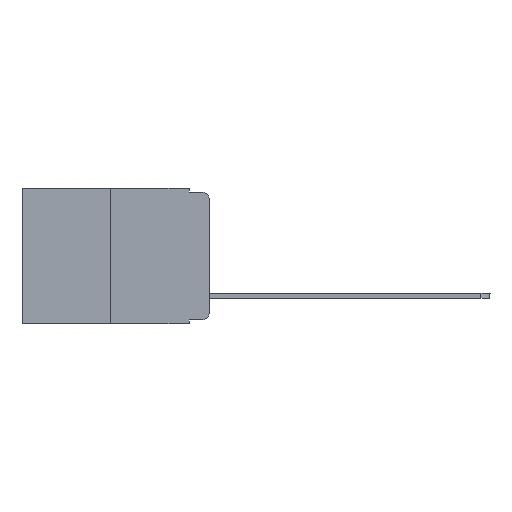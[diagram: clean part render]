
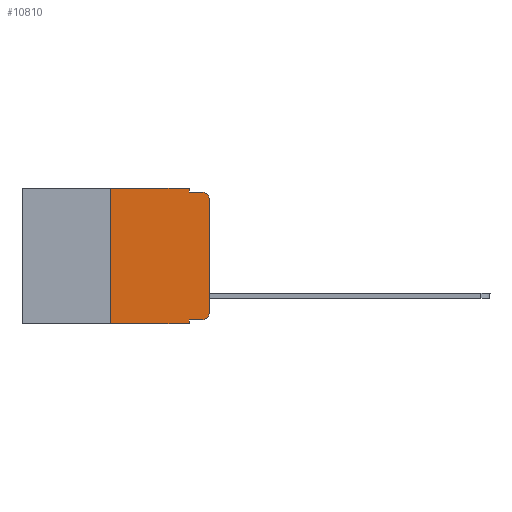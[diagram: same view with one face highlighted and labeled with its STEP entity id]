
A CAD part, left-side view. The second image highlights one B-rep face of the part: STEP entity #10810.
In plain terms, the highlighted planar face has unit normal (-1, 0, 0).
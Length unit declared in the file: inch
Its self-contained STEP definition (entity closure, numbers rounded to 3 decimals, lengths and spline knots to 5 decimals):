
#530 = EDGE_CURVE ( 'NONE', #2004, #8552, #6242, .T. ) ;
#583 = ORIENTED_EDGE ( 'NONE', *, *, #7575, .T. ) ;
#757 = VERTEX_POINT ( 'NONE', #7477 ) ;
#797 = CARTESIAN_POINT ( 'NONE',  ( 0., 0.051, -0.333 ) ) ;
#846 = ORIENTED_EDGE ( 'NONE', *, *, #15394, .F. ) ;
#1060 = LINE ( 'NONE', #16022, #6689 ) ;
#1316 = VERTEX_POINT ( 'NONE', #16605 ) ;
#1617 = EDGE_LOOP ( 'NONE', ( #15454, #12540, #11652, #846, #2508, #5931, #3821, #10729, #14187, #583 ) ) ;
#1690 = EDGE_CURVE ( 'NONE', #13678, #1316, #13811, .T. ) ;
#1739 = CARTESIAN_POINT ( 'NONE',  ( 0., 0.25, 0. ) ) ;
#1798 = DIRECTION ( 'NONE',  ( 0., 0., -1. ) ) ;
#2004 = VERTEX_POINT ( 'NONE', #2805 ) ;
#2341 = DIRECTION ( 'NONE',  ( 0., -1., 0. ) ) ;
#2508 = ORIENTED_EDGE ( 'NONE', *, *, #1690, .F. ) ;
#2805 = CARTESIAN_POINT ( 'NONE',  ( 0., 0.051, -0.01 ) ) ;
#3271 = CARTESIAN_POINT ( 'NONE',  ( 0., 0.051, -0.333 ) ) ;
#3319 = CARTESIAN_POINT ( 'NONE',  ( 0., 0.051, -0.01 ) ) ;
#3321 = LINE ( 'NONE', #7506, #8399 ) ;
#3367 = VERTEX_POINT ( 'NONE', #5402 ) ;
#3459 = VERTEX_POINT ( 'NONE', #9952 ) ;
#3486 = DIRECTION ( 'NONE',  ( 0., -1., 0. ) ) ;
#3665 = CARTESIAN_POINT ( 'NONE',  ( 0., 0.051, -0.343 ) ) ;
#3821 = ORIENTED_EDGE ( 'NONE', *, *, #6751, .T. ) ;
#4002 = CARTESIAN_POINT ( 'NONE',  ( 0., 0.02, -0.01 ) ) ;
#4651 = VECTOR ( 'NONE', #7163, 39.37008 ) ;
#4835 = LINE ( 'NONE', #9129, #12370 ) ;
#4858 = DIRECTION ( 'NONE',  ( -1., 0., 0. ) ) ;
#5402 = CARTESIAN_POINT ( 'NONE',  ( 0., 0., -0.313 ) ) ;
#5602 = DIRECTION ( 'NONE',  ( 0., -1., 0. ) ) ;
#5931 = ORIENTED_EDGE ( 'NONE', *, *, #16670, .F. ) ;
#6012 = VECTOR ( 'NONE', #6200, 39.37008 ) ;
#6200 = DIRECTION ( 'NONE',  ( 0., -1., 0. ) ) ;
#6242 = LINE ( 'NONE', #3319, #7376 ) ;
#6368 = EDGE_CURVE ( 'NONE', #3367, #757, #4835, .T. ) ;
#6689 = VECTOR ( 'NONE', #8980, 39.37008 ) ;
#6751 = EDGE_CURVE ( 'NONE', #3459, #12503, #11690, .T. ) ;
#6963 = AXIS2_PLACEMENT_3D ( 'NONE', #17096, #4858, #10316 ) ;
#7163 = DIRECTION ( 'NONE',  ( 0., 0., 1. ) ) ;
#7376 = VECTOR ( 'NONE', #3486, 39.37008 ) ;
#7390 = PLANE ( 'NONE',  #16487 ) ;
#7477 = CARTESIAN_POINT ( 'NONE',  ( 0., 0., -0.03 ) ) ;
#7506 = CARTESIAN_POINT ( 'NONE',  ( 0., 0.051, 0. ) ) ;
#7575 = EDGE_CURVE ( 'NONE', #11278, #3367, #12357, .T. ) ;
#8399 = VECTOR ( 'NONE', #8846, 39.37008 ) ;
#8497 = VECTOR ( 'NONE', #2341, 39.37008 ) ;
#8552 = VERTEX_POINT ( 'NONE', #4002 ) ;
#8846 = DIRECTION ( 'NONE',  ( 0., 0., -1. ) ) ;
#8980 = DIRECTION ( 'NONE',  ( 0., 0., -1. ) ) ;
#9129 = CARTESIAN_POINT ( 'NONE',  ( 0., 0., 0. ) ) ;
#9565 = CARTESIAN_POINT ( 'NONE',  ( 0., 0.02, -0.03 ) ) ;
#9649 = DIRECTION ( 'NONE',  ( 0., 0., -1. ) ) ;
#9952 = CARTESIAN_POINT ( 'NONE',  ( 0., 0.25, -0.343 ) ) ;
#9993 = VERTEX_POINT ( 'NONE', #3271 ) ;
#10131 = CARTESIAN_POINT ( 'NONE',  ( 0., 0.02, -0.333 ) ) ;
#10316 = DIRECTION ( 'NONE',  ( 0., 0., -1. ) ) ;
#10729 = ORIENTED_EDGE ( 'NONE', *, *, #11468, .F. ) ;
#10810 = ADVANCED_FACE ( 'NONE', ( #15511 ), #7390, .F. ) ;
#11278 = VERTEX_POINT ( 'NONE', #10131 ) ;
#11468 = EDGE_CURVE ( 'NONE', #9993, #12503, #1060, .T. ) ;
#11494 = CARTESIAN_POINT ( 'NONE',  ( 0., 0.473, 0. ) ) ;
#11612 = CARTESIAN_POINT ( 'NONE',  ( 0., 0.473, -0.343 ) ) ;
#11652 = ORIENTED_EDGE ( 'NONE', *, *, #530, .F. ) ;
#11690 = LINE ( 'NONE', #11612, #8497 ) ;
#12357 = CIRCLE ( 'NONE', #6963, 0.02 ) ;
#12370 = VECTOR ( 'NONE', #17166, 39.37008 ) ;
#12503 = VERTEX_POINT ( 'NONE', #3665 ) ;
#12540 = ORIENTED_EDGE ( 'NONE', *, *, #17425, .T. ) ;
#13150 = LINE ( 'NONE', #797, #6012 ) ;
#13524 = EDGE_CURVE ( 'NONE', #9993, #11278, #13150, .T. ) ;
#13678 = VERTEX_POINT ( 'NONE', #14777 ) ;
#13713 = CARTESIAN_POINT ( 'NONE',  ( 0., 0.473, 0. ) ) ;
#13796 = AXIS2_PLACEMENT_3D ( 'NONE', #9565, #15014, #9649 ) ;
#13811 = LINE ( 'NONE', #13713, #15112 ) ;
#13991 = DIRECTION ( 'NONE',  ( 1., 0., 0. ) ) ;
#14187 = ORIENTED_EDGE ( 'NONE', *, *, #13524, .T. ) ;
#14200 = LINE ( 'NONE', #1739, #4651 ) ;
#14777 = CARTESIAN_POINT ( 'NONE',  ( 0., 0.25, 0. ) ) ;
#15014 = DIRECTION ( 'NONE',  ( -1., 0., 0. ) ) ;
#15112 = VECTOR ( 'NONE', #5602, 39.37008 ) ;
#15394 = EDGE_CURVE ( 'NONE', #1316, #2004, #3321, .T. ) ;
#15454 = ORIENTED_EDGE ( 'NONE', *, *, #6368, .T. ) ;
#15511 = FACE_OUTER_BOUND ( 'NONE', #1617, .T. ) ;
#16022 = CARTESIAN_POINT ( 'NONE',  ( 0., 0.051, 0. ) ) ;
#16378 = CIRCLE ( 'NONE', #13796, 0.02 ) ;
#16487 = AXIS2_PLACEMENT_3D ( 'NONE', #11494, #13991, #1798 ) ;
#16605 = CARTESIAN_POINT ( 'NONE',  ( 0., 0.051, 0. ) ) ;
#16670 = EDGE_CURVE ( 'NONE', #3459, #13678, #14200, .T. ) ;
#17096 = CARTESIAN_POINT ( 'NONE',  ( 0., 0.02, -0.313 ) ) ;
#17166 = DIRECTION ( 'NONE',  ( 0., 0., 1. ) ) ;
#17425 = EDGE_CURVE ( 'NONE', #757, #8552, #16378, .T. ) ;
